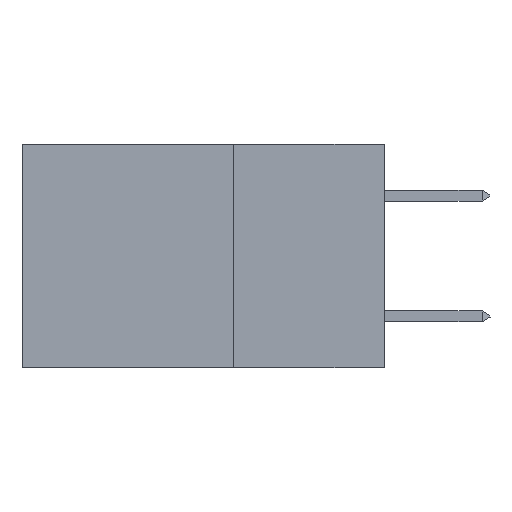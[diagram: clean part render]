
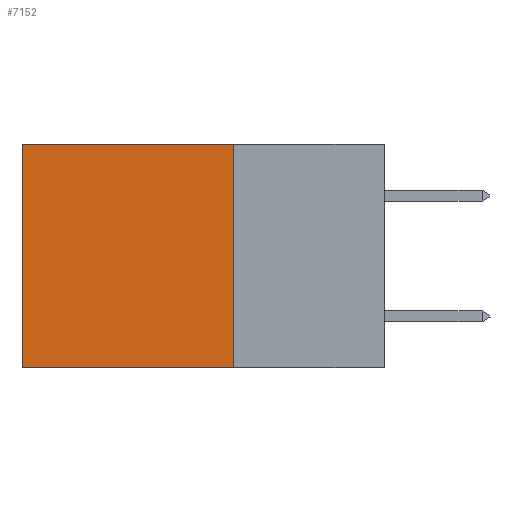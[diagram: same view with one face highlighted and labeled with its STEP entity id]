
A CAD part, left-side view. The second image highlights one B-rep face of the part: STEP entity #7152.
In plain terms, the highlighted planar face has unit normal (-1, 0, 0).
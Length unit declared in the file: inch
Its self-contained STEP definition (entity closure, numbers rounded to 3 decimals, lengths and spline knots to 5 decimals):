
#3250 = CARTESIAN_POINT ( 'NONE',  ( 0.2875, 0.25, 0. ) ) ;
#3567 = VECTOR ( 'NONE', #35072, 39.37008 ) ;
#6365 = VERTEX_POINT ( 'NONE', #17612 ) ;
#7152 = ADVANCED_FACE ( 'NONE', ( #42123 ), #9346, .F. ) ;
#8991 = CARTESIAN_POINT ( 'NONE',  ( 0.2875, 0.25, -0.37 ) ) ;
#9346 = PLANE ( 'NONE',  #21887 ) ;
#11038 = LINE ( 'NONE', #21161, #16480 ) ;
#11527 = VERTEX_POINT ( 'NONE', #16826 ) ;
#11654 = LINE ( 'NONE', #21565, #20872 ) ;
#12725 = VERTEX_POINT ( 'NONE', #25477 ) ;
#15100 = EDGE_CURVE ( 'NONE', #21315, #6365, #11038, .T. ) ;
#15126 = DIRECTION ( 'NONE',  ( 0., 1., 0. ) ) ;
#16480 = VECTOR ( 'NONE', #15126, 39.37008 ) ;
#16826 = CARTESIAN_POINT ( 'NONE',  ( 0.2875, 0.25, -0.37 ) ) ;
#17612 = CARTESIAN_POINT ( 'NONE',  ( 0.2875, 0.6, 0. ) ) ;
#18556 = LINE ( 'NONE', #24597, #31201 ) ;
#18700 = LINE ( 'NONE', #8991, #3567 ) ;
#20872 = VECTOR ( 'NONE', #34286, 39.37008 ) ;
#21161 = CARTESIAN_POINT ( 'NONE',  ( 0.2875, 0.25, 0. ) ) ;
#21315 = VERTEX_POINT ( 'NONE', #3250 ) ;
#21565 = CARTESIAN_POINT ( 'NONE',  ( 0.2875, 0.25, 0. ) ) ;
#21887 = AXIS2_PLACEMENT_3D ( 'NONE', #22482, #25947, #39091 ) ;
#22482 = CARTESIAN_POINT ( 'NONE',  ( 0.2875, 0.25, 0. ) ) ;
#23474 = EDGE_LOOP ( 'NONE', ( #29096, #24846, #36765, #35154 ) ) ;
#24597 = CARTESIAN_POINT ( 'NONE',  ( 0.2875, 0.6, 0. ) ) ;
#24846 = ORIENTED_EDGE ( 'NONE', *, *, #39689, .F. ) ;
#25477 = CARTESIAN_POINT ( 'NONE',  ( 0.2875, 0.6, -0.37 ) ) ;
#25947 = DIRECTION ( 'NONE',  ( 1., 0., 0. ) ) ;
#29096 = ORIENTED_EDGE ( 'NONE', *, *, #42528, .T. ) ;
#31201 = VECTOR ( 'NONE', #37742, 39.37008 ) ;
#34286 = DIRECTION ( 'NONE',  ( 0., 0., -1. ) ) ;
#35072 = DIRECTION ( 'NONE',  ( 0., 1., 0. ) ) ;
#35154 = ORIENTED_EDGE ( 'NONE', *, *, #15100, .T. ) ;
#36765 = ORIENTED_EDGE ( 'NONE', *, *, #40550, .F. ) ;
#37742 = DIRECTION ( 'NONE',  ( 0., 0., -1. ) ) ;
#39091 = DIRECTION ( 'NONE',  ( 0., 0., -1. ) ) ;
#39689 = EDGE_CURVE ( 'NONE', #11527, #12725, #18700, .T. ) ;
#40550 = EDGE_CURVE ( 'NONE', #21315, #11527, #11654, .T. ) ;
#42123 = FACE_OUTER_BOUND ( 'NONE', #23474, .T. ) ;
#42528 = EDGE_CURVE ( 'NONE', #6365, #12725, #18556, .T. ) ;
